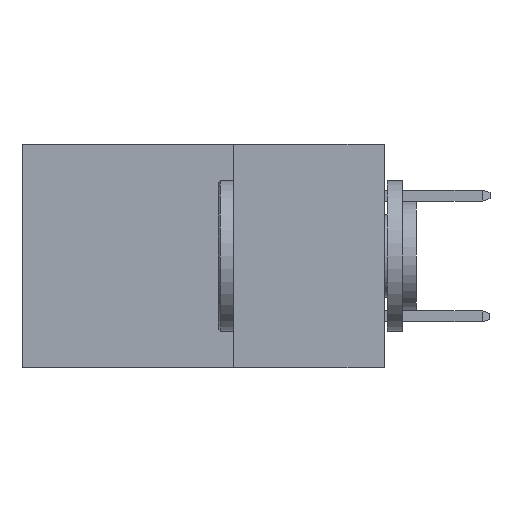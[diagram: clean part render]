
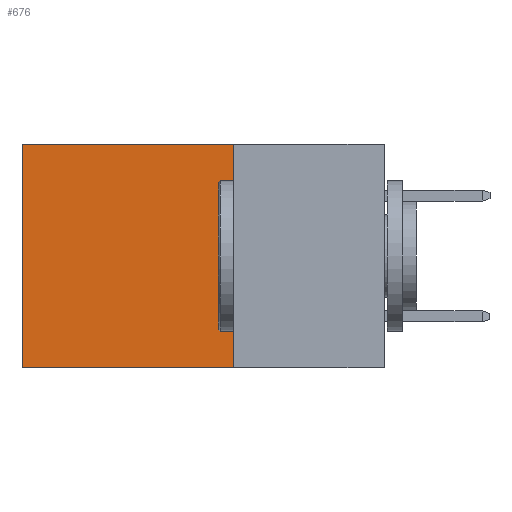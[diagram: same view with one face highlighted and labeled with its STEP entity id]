
A CAD part, left-side view. The second image highlights one B-rep face of the part: STEP entity #676.
In plain terms, the highlighted planar face has unit normal (-1, 0, 0).
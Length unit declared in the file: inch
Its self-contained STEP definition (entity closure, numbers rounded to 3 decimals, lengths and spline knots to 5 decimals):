
#676 = ADVANCED_FACE ( 'NONE', ( #12687 ), #10547, .F. ) ;
#774 = CARTESIAN_POINT ( 'NONE',  ( 0.298, 0.25, -0.37 ) ) ;
#930 = EDGE_LOOP ( 'NONE', ( #6547, #6892, #10061, #10379 ) ) ;
#933 = LINE ( 'NONE', #774, #1277 ) ;
#1277 = VECTOR ( 'NONE', #7275, 39.37008 ) ;
#1581 = VECTOR ( 'NONE', #11553, 39.37008 ) ;
#1744 = VERTEX_POINT ( 'NONE', #8350 ) ;
#1802 = CARTESIAN_POINT ( 'NONE',  ( 0.298, 0.25, 0. ) ) ;
#3263 = VERTEX_POINT ( 'NONE', #8418 ) ;
#3634 = DIRECTION ( 'NONE',  ( 0., 0., -1. ) ) ;
#3859 = DIRECTION ( 'NONE',  ( 0., 0., -1. ) ) ;
#3867 = DIRECTION ( 'NONE',  ( 1., 0., 0. ) ) ;
#4372 = CARTESIAN_POINT ( 'NONE',  ( 0.298, 0.25, 0. ) ) ;
#4410 = AXIS2_PLACEMENT_3D ( 'NONE', #4372, #3867, #3859 ) ;
#4823 = EDGE_CURVE ( 'NONE', #1744, #5510, #933, .T. ) ;
#5510 = VERTEX_POINT ( 'NONE', #13500 ) ;
#5577 = VECTOR ( 'NONE', #13635, 39.37008 ) ;
#6076 = VERTEX_POINT ( 'NONE', #6996 ) ;
#6547 = ORIENTED_EDGE ( 'NONE', *, *, #11575, .T. ) ;
#6892 = ORIENTED_EDGE ( 'NONE', *, *, #4823, .F. ) ;
#6996 = CARTESIAN_POINT ( 'NONE',  ( 0.298, 0.6, 0. ) ) ;
#7189 = EDGE_CURVE ( 'NONE', #3263, #6076, #11251, .T. ) ;
#7275 = DIRECTION ( 'NONE',  ( 0., 1., 0. ) ) ;
#8311 = LINE ( 'NONE', #10152, #13834 ) ;
#8350 = CARTESIAN_POINT ( 'NONE',  ( 0.298, 0.25, -0.37 ) ) ;
#8418 = CARTESIAN_POINT ( 'NONE',  ( 0.298, 0.25, 0. ) ) ;
#10061 = ORIENTED_EDGE ( 'NONE', *, *, #13886, .F. ) ;
#10152 = CARTESIAN_POINT ( 'NONE',  ( 0.298, 0.6, 0. ) ) ;
#10299 = LINE ( 'NONE', #10502, #1581 ) ;
#10379 = ORIENTED_EDGE ( 'NONE', *, *, #7189, .T. ) ;
#10502 = CARTESIAN_POINT ( 'NONE',  ( 0.298, 0.25, 0. ) ) ;
#10547 = PLANE ( 'NONE',  #4410 ) ;
#11251 = LINE ( 'NONE', #1802, #5577 ) ;
#11553 = DIRECTION ( 'NONE',  ( 0., 0., -1. ) ) ;
#11575 = EDGE_CURVE ( 'NONE', #6076, #5510, #8311, .T. ) ;
#12687 = FACE_OUTER_BOUND ( 'NONE', #930, .T. ) ;
#13500 = CARTESIAN_POINT ( 'NONE',  ( 0.298, 0.6, -0.37 ) ) ;
#13635 = DIRECTION ( 'NONE',  ( 0., 1., 0. ) ) ;
#13834 = VECTOR ( 'NONE', #3634, 39.37008 ) ;
#13886 = EDGE_CURVE ( 'NONE', #3263, #1744, #10299, .T. ) ;
